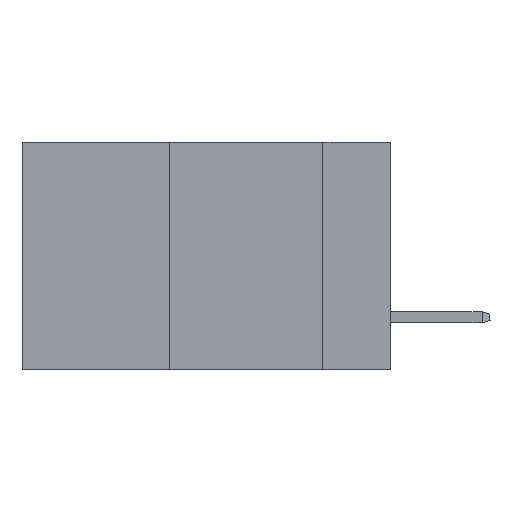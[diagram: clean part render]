
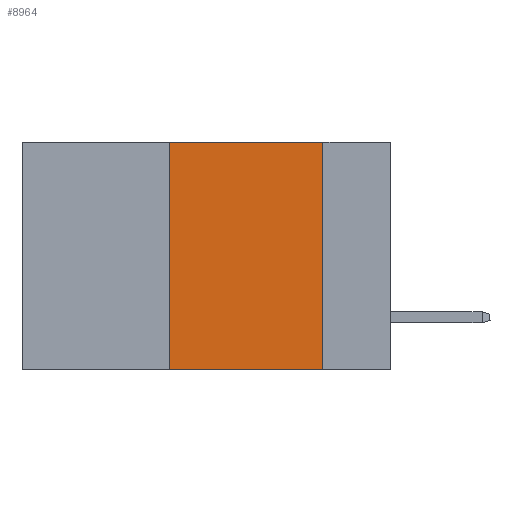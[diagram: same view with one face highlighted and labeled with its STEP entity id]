
A CAD part, left-side view. The second image highlights one B-rep face of the part: STEP entity #8964.
In plain terms, the highlighted planar face has unit normal (-1, 0, 0).
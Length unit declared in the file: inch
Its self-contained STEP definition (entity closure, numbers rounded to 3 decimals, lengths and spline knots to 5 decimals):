
#297 = VECTOR ( 'NONE', #4935, 39.37008 ) ;
#833 = VERTEX_POINT ( 'NONE', #7127 ) ;
#1062 = FACE_OUTER_BOUND ( 'NONE', #5581, .T. ) ;
#1390 = LINE ( 'NONE', #3880, #4113 ) ;
#1539 = CARTESIAN_POINT ( 'NONE',  ( 0., 0.11, 0. ) ) ;
#1842 = ORIENTED_EDGE ( 'NONE', *, *, #2135, .T. ) ;
#2109 = DIRECTION ( 'NONE',  ( 0., 0., -1. ) ) ;
#2135 = EDGE_CURVE ( 'NONE', #14654, #4996, #6651, .T. ) ;
#2670 = DIRECTION ( 'NONE',  ( 0., -1., 0. ) ) ;
#3409 = CARTESIAN_POINT ( 'NONE',  ( 0., 0.36, 0. ) ) ;
#3880 = CARTESIAN_POINT ( 'NONE',  ( 0., 0.6, 0. ) ) ;
#3923 = AXIS2_PLACEMENT_3D ( 'NONE', #8012, #11622, #2109 ) ;
#4113 = VECTOR ( 'NONE', #2670, 39.37008 ) ;
#4521 = PLANE ( 'NONE',  #3923 ) ;
#4935 = DIRECTION ( 'NONE',  ( 0., 0., -1. ) ) ;
#4996 = VERTEX_POINT ( 'NONE', #7104 ) ;
#5369 = DIRECTION ( 'NONE',  ( 0., -1., 0. ) ) ;
#5450 = EDGE_CURVE ( 'NONE', #833, #9871, #1390, .T. ) ;
#5581 = EDGE_LOOP ( 'NONE', ( #13720, #11939, #6967, #1842 ) ) ;
#5965 = VECTOR ( 'NONE', #5369, 39.37008 ) ;
#6651 = LINE ( 'NONE', #10973, #5965 ) ;
#6967 = ORIENTED_EDGE ( 'NONE', *, *, #8601, .F. ) ;
#7104 = CARTESIAN_POINT ( 'NONE',  ( 0., 0.11, -0.37 ) ) ;
#7127 = CARTESIAN_POINT ( 'NONE',  ( 0., 0.36, 0. ) ) ;
#8012 = CARTESIAN_POINT ( 'NONE',  ( 0., 0.6, 0. ) ) ;
#8344 = LINE ( 'NONE', #1539, #297 ) ;
#8601 = EDGE_CURVE ( 'NONE', #14654, #833, #13767, .T. ) ;
#8964 = ADVANCED_FACE ( 'NONE', ( #1062 ), #4521, .F. ) ;
#9871 = VERTEX_POINT ( 'NONE', #11105 ) ;
#10373 = DIRECTION ( 'NONE',  ( 0., 0., 1. ) ) ;
#10973 = CARTESIAN_POINT ( 'NONE',  ( 0., 0.6, -0.37 ) ) ;
#11105 = CARTESIAN_POINT ( 'NONE',  ( 0., 0.11, 0. ) ) ;
#11622 = DIRECTION ( 'NONE',  ( 1., 0., 0. ) ) ;
#11939 = ORIENTED_EDGE ( 'NONE', *, *, #5450, .F. ) ;
#12272 = CARTESIAN_POINT ( 'NONE',  ( 0., 0.36, -0.37 ) ) ;
#12598 = VECTOR ( 'NONE', #10373, 39.37008 ) ;
#13720 = ORIENTED_EDGE ( 'NONE', *, *, #14582, .F. ) ;
#13767 = LINE ( 'NONE', #3409, #12598 ) ;
#14582 = EDGE_CURVE ( 'NONE', #9871, #4996, #8344, .T. ) ;
#14654 = VERTEX_POINT ( 'NONE', #12272 ) ;
